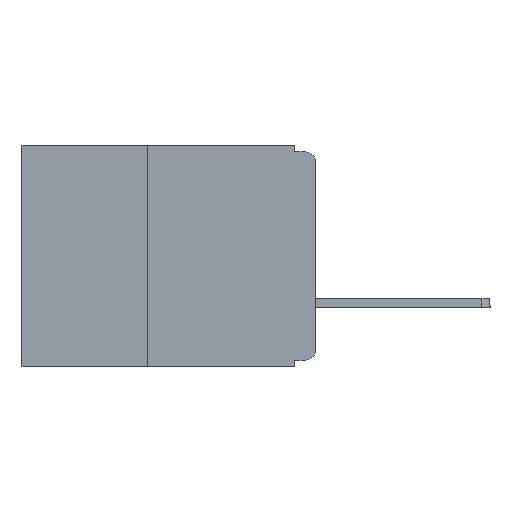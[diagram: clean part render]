
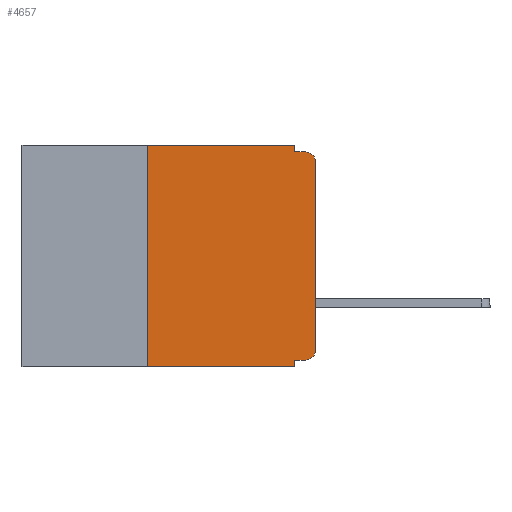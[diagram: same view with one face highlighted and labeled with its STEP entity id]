
A CAD part, left-side view. The second image highlights one B-rep face of the part: STEP entity #4657.
In plain terms, the highlighted planar face has unit normal (-1, 0, 0).
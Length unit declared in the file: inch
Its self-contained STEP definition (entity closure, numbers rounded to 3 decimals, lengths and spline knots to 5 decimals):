
#614 = VERTEX_POINT ( 'NONE', #14927 ) ;
#666 = CARTESIAN_POINT ( 'NONE',  ( 0., 0.25, -0.33 ) ) ;
#763 = VECTOR ( 'NONE', #31229, 39.37008 ) ;
#1116 = VECTOR ( 'NONE', #31190, 39.37008 ) ;
#1271 = LINE ( 'NONE', #3428, #20045 ) ;
#1489 = ORIENTED_EDGE ( 'NONE', *, *, #23466, .T. ) ;
#1660 = CARTESIAN_POINT ( 'NONE',  ( 0., 0.015, -0.32 ) ) ;
#1814 = CARTESIAN_POINT ( 'NONE',  ( 0., 0.031, -0.32 ) ) ;
#1913 = VERTEX_POINT ( 'NONE', #1660 ) ;
#2010 = ORIENTED_EDGE ( 'NONE', *, *, #15338, .F. ) ;
#2051 = CARTESIAN_POINT ( 'NONE',  ( 0., 0.015, -0.305 ) ) ;
#2500 = DIRECTION ( 'NONE',  ( 0., -1., 0. ) ) ;
#2740 = VERTEX_POINT ( 'NONE', #29096 ) ;
#2769 = CARTESIAN_POINT ( 'NONE',  ( 0., 0., 0. ) ) ;
#2875 = VERTEX_POINT ( 'NONE', #25419 ) ;
#3428 = CARTESIAN_POINT ( 'NONE',  ( 0., 0.031, -0.33 ) ) ;
#3619 = EDGE_LOOP ( 'NONE', ( #25478, #10903, #26938, #18328, #22597, #2010, #22554, #18246, #12698, #1489 ) ) ;
#4613 = DIRECTION ( 'NONE',  ( 0., 0., -1. ) ) ;
#4657 = ADVANCED_FACE ( 'NONE', ( #6417 ), #15010, .F. ) ;
#4769 = VERTEX_POINT ( 'NONE', #12397 ) ;
#5428 = VECTOR ( 'NONE', #2500, 39.37008 ) ;
#5766 = CARTESIAN_POINT ( 'NONE',  ( 0., 0., -0.01 ) ) ;
#5842 = CARTESIAN_POINT ( 'NONE',  ( 0., 0.031, 0. ) ) ;
#6015 = DIRECTION ( 'NONE',  ( 0., 0., -1. ) ) ;
#6417 = FACE_OUTER_BOUND ( 'NONE', #3619, .T. ) ;
#7563 = LINE ( 'NONE', #5842, #763 ) ;
#8068 = CARTESIAN_POINT ( 'NONE',  ( 0., 0., -0.32 ) ) ;
#8292 = VERTEX_POINT ( 'NONE', #13111 ) ;
#8438 = CARTESIAN_POINT ( 'NONE',  ( 0., 0.015, -0.025 ) ) ;
#8514 = CARTESIAN_POINT ( 'NONE',  ( 0., 0.015, -0.01 ) ) ;
#8901 = EDGE_CURVE ( 'NONE', #1913, #27719, #11120, .T. ) ;
#9692 = CARTESIAN_POINT ( 'NONE',  ( 0., 0., -0.025 ) ) ;
#9914 = EDGE_CURVE ( 'NONE', #4769, #8292, #32408, .T. ) ;
#9983 = CIRCLE ( 'NONE', #26375, 0.015 ) ;
#10143 = EDGE_CURVE ( 'NONE', #13754, #26373, #20992, .T. ) ;
#10903 = ORIENTED_EDGE ( 'NONE', *, *, #10143, .T. ) ;
#11004 = DIRECTION ( 'NONE',  ( 0., 0., -1. ) ) ;
#11120 = LINE ( 'NONE', #8068, #11899 ) ;
#11297 = VECTOR ( 'NONE', #23593, 39.37008 ) ;
#11392 = VECTOR ( 'NONE', #13037, 39.37008 ) ;
#11899 = VECTOR ( 'NONE', #25855, 39.37008 ) ;
#12055 = DIRECTION ( 'NONE',  ( 0., -1., 0. ) ) ;
#12177 = LINE ( 'NONE', #2769, #11392 ) ;
#12292 = EDGE_CURVE ( 'NONE', #27719, #8292, #1271, .T. ) ;
#12397 = CARTESIAN_POINT ( 'NONE',  ( 0., 0.25, -0.33 ) ) ;
#12698 = ORIENTED_EDGE ( 'NONE', *, *, #8901, .F. ) ;
#13037 = DIRECTION ( 'NONE',  ( 0., 0., 1. ) ) ;
#13111 = CARTESIAN_POINT ( 'NONE',  ( 0., 0.031, -0.33 ) ) ;
#13754 = VERTEX_POINT ( 'NONE', #9692 ) ;
#14447 = AXIS2_PLACEMENT_3D ( 'NONE', #8438, #26220, #11004 ) ;
#14662 = LINE ( 'NONE', #666, #1116 ) ;
#14665 = EDGE_CURVE ( 'NONE', #614, #31378, #7563, .T. ) ;
#14927 = CARTESIAN_POINT ( 'NONE',  ( 0., 0.031, 0. ) ) ;
#14936 = DIRECTION ( 'NONE',  ( 0., 0., -1. ) ) ;
#14967 = DIRECTION ( 'NONE',  ( 1., 0., 0. ) ) ;
#15010 = PLANE ( 'NONE',  #20959 ) ;
#15103 = CARTESIAN_POINT ( 'NONE',  ( 0., 0.031, -0.01 ) ) ;
#15338 = EDGE_CURVE ( 'NONE', #4769, #2740, #14662, .T. ) ;
#15446 = CARTESIAN_POINT ( 'NONE',  ( 0., 0.437, 0. ) ) ;
#18246 = ORIENTED_EDGE ( 'NONE', *, *, #12292, .F. ) ;
#18328 = ORIENTED_EDGE ( 'NONE', *, *, #14665, .F. ) ;
#19645 = CARTESIAN_POINT ( 'NONE',  ( 0., 0.437, 0. ) ) ;
#19923 = DIRECTION ( 'NONE',  ( -1., 0., 0. ) ) ;
#20045 = VECTOR ( 'NONE', #6015, 39.37008 ) ;
#20665 = EDGE_CURVE ( 'NONE', #2875, #13754, #12177, .T. ) ;
#20959 = AXIS2_PLACEMENT_3D ( 'NONE', #15446, #14967, #14936 ) ;
#20992 = CIRCLE ( 'NONE', #14447, 0.015 ) ;
#22554 = ORIENTED_EDGE ( 'NONE', *, *, #9914, .T. ) ;
#22597 = ORIENTED_EDGE ( 'NONE', *, *, #26613, .F. ) ;
#23466 = EDGE_CURVE ( 'NONE', #1913, #2875, #9983, .T. ) ;
#23593 = DIRECTION ( 'NONE',  ( 0., -1., 0. ) ) ;
#25419 = CARTESIAN_POINT ( 'NONE',  ( 0., 0., -0.305 ) ) ;
#25478 = ORIENTED_EDGE ( 'NONE', *, *, #20665, .T. ) ;
#25855 = DIRECTION ( 'NONE',  ( 0., 1., 0. ) ) ;
#26220 = DIRECTION ( 'NONE',  ( -1., 0., 0. ) ) ;
#26373 = VERTEX_POINT ( 'NONE', #8514 ) ;
#26375 = AXIS2_PLACEMENT_3D ( 'NONE', #2051, #19923, #4613 ) ;
#26613 = EDGE_CURVE ( 'NONE', #2740, #614, #29222, .T. ) ;
#26938 = ORIENTED_EDGE ( 'NONE', *, *, #27842, .F. ) ;
#27719 = VERTEX_POINT ( 'NONE', #1814 ) ;
#27842 = EDGE_CURVE ( 'NONE', #31378, #26373, #29894, .T. ) ;
#27866 = CARTESIAN_POINT ( 'NONE',  ( 0., 0.437, -0.33 ) ) ;
#28431 = VECTOR ( 'NONE', #12055, 39.37008 ) ;
#29096 = CARTESIAN_POINT ( 'NONE',  ( 0., 0.25, 0. ) ) ;
#29222 = LINE ( 'NONE', #19645, #28431 ) ;
#29894 = LINE ( 'NONE', #5766, #11297 ) ;
#31190 = DIRECTION ( 'NONE',  ( 0., 0., 1. ) ) ;
#31229 = DIRECTION ( 'NONE',  ( 0., 0., -1. ) ) ;
#31378 = VERTEX_POINT ( 'NONE', #15103 ) ;
#32408 = LINE ( 'NONE', #27866, #5428 ) ;
